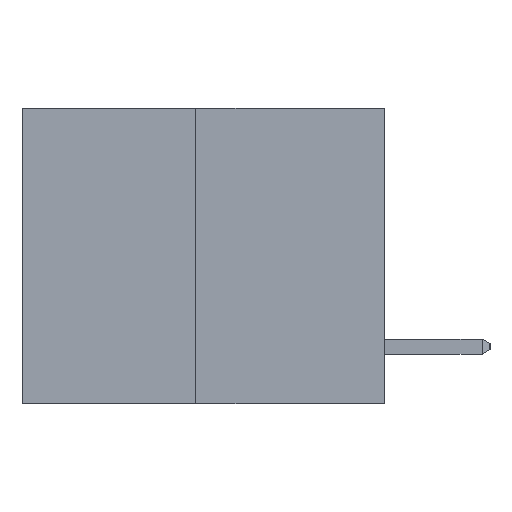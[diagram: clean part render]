
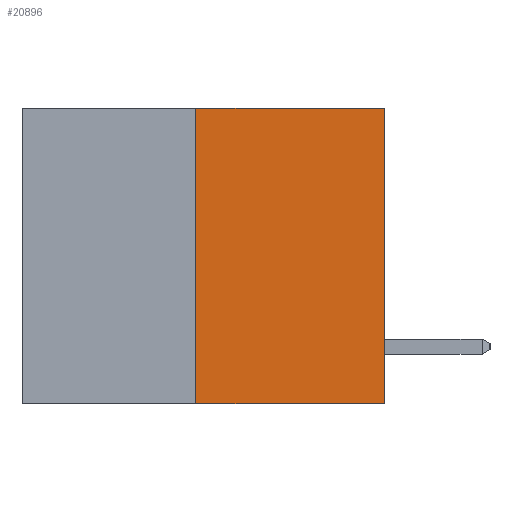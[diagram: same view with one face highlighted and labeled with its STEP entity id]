
A CAD part, left-side view. The second image highlights one B-rep face of the part: STEP entity #20896.
In plain terms, the highlighted planar face has unit normal (-1, 0, 0).
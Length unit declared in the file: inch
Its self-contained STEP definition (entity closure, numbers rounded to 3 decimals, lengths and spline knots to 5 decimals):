
#1178 = CARTESIAN_POINT ( 'NONE',  ( 0., 0.6, 0. ) ) ;
#1359 = CARTESIAN_POINT ( 'NONE',  ( 0., 0.6, 0. ) ) ;
#1570 = FACE_OUTER_BOUND ( 'NONE', #13324, .T. ) ;
#3095 = DIRECTION ( 'NONE',  ( 0., 0., 1. ) ) ;
#3416 = DIRECTION ( 'NONE',  ( 0., 0., -1. ) ) ;
#3653 = DIRECTION ( 'NONE',  ( 0., -1., 0. ) ) ;
#4642 = CARTESIAN_POINT ( 'NONE',  ( 0., 0.312, -0.49 ) ) ;
#4870 = VERTEX_POINT ( 'NONE', #8172 ) ;
#5049 = LINE ( 'NONE', #1178, #11311 ) ;
#5613 = DIRECTION ( 'NONE',  ( 0., 0., 1. ) ) ;
#5672 = LINE ( 'NONE', #14022, #21847 ) ;
#7239 = ORIENTED_EDGE ( 'NONE', *, *, #22085, .F. ) ;
#7903 = VERTEX_POINT ( 'NONE', #8460 ) ;
#8172 = CARTESIAN_POINT ( 'NONE',  ( 0., 0.312, 0. ) ) ;
#8428 = DIRECTION ( 'NONE',  ( 0., -1., 0. ) ) ;
#8460 = CARTESIAN_POINT ( 'NONE',  ( 0., 0., -0.49 ) ) ;
#9178 = VERTEX_POINT ( 'NONE', #4642 ) ;
#11311 = VECTOR ( 'NONE', #8428, 39.37008 ) ;
#12560 = CARTESIAN_POINT ( 'NONE',  ( 0., 0., 0. ) ) ;
#12657 = EDGE_CURVE ( 'NONE', #9178, #7903, #12851, .T. ) ;
#12851 = LINE ( 'NONE', #14547, #20184 ) ;
#13324 = EDGE_LOOP ( 'NONE', ( #19153, #23097, #14019, #7239 ) ) ;
#13631 = EDGE_CURVE ( 'NONE', #9178, #4870, #20138, .T. ) ;
#13856 = EDGE_CURVE ( 'NONE', #7903, #16677, #5672, .T. ) ;
#14019 = ORIENTED_EDGE ( 'NONE', *, *, #13856, .T. ) ;
#14022 = CARTESIAN_POINT ( 'NONE',  ( 0., 0., 0. ) ) ;
#14547 = CARTESIAN_POINT ( 'NONE',  ( 0., 0.6, -0.49 ) ) ;
#15937 = PLANE ( 'NONE',  #19093 ) ;
#16677 = VERTEX_POINT ( 'NONE', #12560 ) ;
#17679 = DIRECTION ( 'NONE',  ( 1., 0., 0. ) ) ;
#18250 = CARTESIAN_POINT ( 'NONE',  ( 0., 0.312, -0.49 ) ) ;
#19093 = AXIS2_PLACEMENT_3D ( 'NONE', #1359, #17679, #3416 ) ;
#19153 = ORIENTED_EDGE ( 'NONE', *, *, #13631, .F. ) ;
#20138 = LINE ( 'NONE', #18250, #22140 ) ;
#20184 = VECTOR ( 'NONE', #3653, 39.37008 ) ;
#20896 = ADVANCED_FACE ( 'NONE', ( #1570 ), #15937, .F. ) ;
#21847 = VECTOR ( 'NONE', #3095, 39.37008 ) ;
#22085 = EDGE_CURVE ( 'NONE', #4870, #16677, #5049, .T. ) ;
#22140 = VECTOR ( 'NONE', #5613, 39.37008 ) ;
#23097 = ORIENTED_EDGE ( 'NONE', *, *, #12657, .T. ) ;
